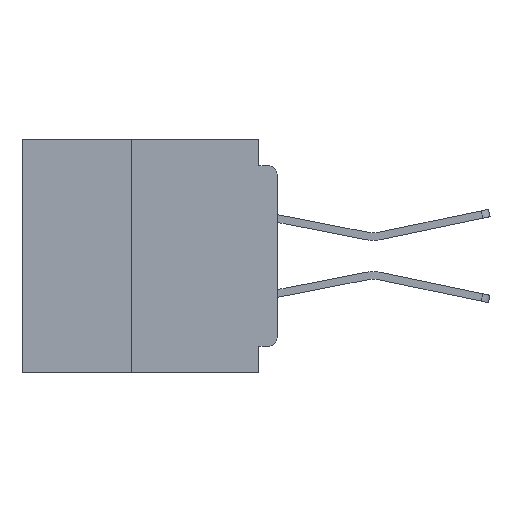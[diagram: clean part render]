
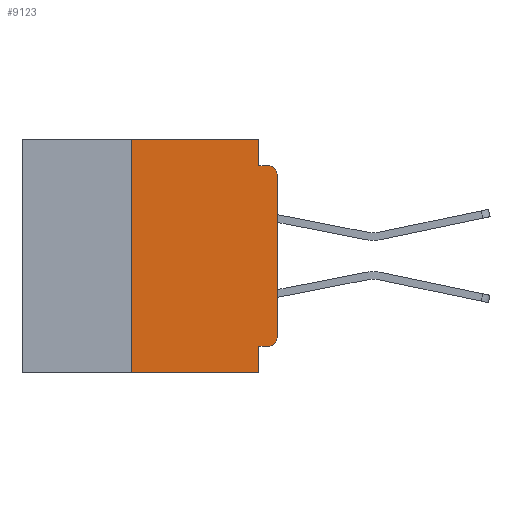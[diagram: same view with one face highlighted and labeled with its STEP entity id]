
A CAD part, left-side view. The second image highlights one B-rep face of the part: STEP entity #9123.
In plain terms, the highlighted planar face has unit normal (-1, 0, 0).
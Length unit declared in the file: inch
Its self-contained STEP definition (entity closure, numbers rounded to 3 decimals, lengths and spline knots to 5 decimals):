
#565 = VECTOR ( 'NONE', #24022, 39.37008 ) ;
#950 = EDGE_CURVE ( 'NONE', #38986, #4719, #29150, .T. ) ;
#1031 = CARTESIAN_POINT ( 'NONE',  ( 0., 0., -0.06 ) ) ;
#1445 = VECTOR ( 'NONE', #38640, 39.37008 ) ;
#2220 = VERTEX_POINT ( 'NONE', #16626 ) ;
#2329 = DIRECTION ( 'NONE',  ( 0., 0., -1. ) ) ;
#2563 = EDGE_CURVE ( 'NONE', #38383, #30484, #29532, .T. ) ;
#2853 = VECTOR ( 'NONE', #5867, 39.37008 ) ;
#4082 = EDGE_CURVE ( 'NONE', #17019, #30484, #7110, .T. ) ;
#4089 = VERTEX_POINT ( 'NONE', #6760 ) ;
#4719 = VERTEX_POINT ( 'NONE', #31256 ) ;
#5179 = CARTESIAN_POINT ( 'NONE',  ( 0., 0.25, -0.4 ) ) ;
#5496 = ORIENTED_EDGE ( 'NONE', *, *, #950, .T. ) ;
#5560 = VERTEX_POINT ( 'NONE', #18147 ) ;
#5867 = DIRECTION ( 'NONE',  ( 0., -1., 0. ) ) ;
#6497 = DIRECTION ( 'NONE',  ( 0., -1., 0. ) ) ;
#6699 = CARTESIAN_POINT ( 'NONE',  ( 0., 0., -0.045 ) ) ;
#6760 = CARTESIAN_POINT ( 'NONE',  ( 0., 0.015, -0.355 ) ) ;
#7110 = LINE ( 'NONE', #6699, #43730 ) ;
#7145 = ORIENTED_EDGE ( 'NONE', *, *, #4082, .F. ) ;
#8577 = ORIENTED_EDGE ( 'NONE', *, *, #44656, .F. ) ;
#9123 = ADVANCED_FACE ( 'NONE', ( #24068 ), #20915, .F. ) ;
#10241 = VECTOR ( 'NONE', #29576, 39.37008 ) ;
#11202 = CARTESIAN_POINT ( 'NONE',  ( 0., 0.031, -0.355 ) ) ;
#12438 = ORIENTED_EDGE ( 'NONE', *, *, #2563, .T. ) ;
#12932 = EDGE_CURVE ( 'NONE', #38986, #5560, #39465, .T. ) ;
#13228 = CARTESIAN_POINT ( 'NONE',  ( 0., 0.437, -0.4 ) ) ;
#13434 = CARTESIAN_POINT ( 'NONE',  ( 0., 0., 0. ) ) ;
#15357 = EDGE_CURVE ( 'NONE', #24697, #17019, #21614, .T. ) ;
#16626 = CARTESIAN_POINT ( 'NONE',  ( 0., 0., -0.34 ) ) ;
#16861 = ORIENTED_EDGE ( 'NONE', *, *, #28020, .T. ) ;
#16980 = EDGE_CURVE ( 'NONE', #4089, #44784, #19795, .T. ) ;
#17019 = VERTEX_POINT ( 'NONE', #43849 ) ;
#17351 = ORIENTED_EDGE ( 'NONE', *, *, #15357, .F. ) ;
#18147 = CARTESIAN_POINT ( 'NONE',  ( 0., 0.25, 0. ) ) ;
#18419 = CIRCLE ( 'NONE', #35934, 0.015 ) ;
#19558 = VECTOR ( 'NONE', #20291, 39.37008 ) ;
#19611 = EDGE_CURVE ( 'NONE', #5560, #24697, #29051, .T. ) ;
#19795 = LINE ( 'NONE', #22295, #10241 ) ;
#20291 = DIRECTION ( 'NONE',  ( 0., 0., 1. ) ) ;
#20442 = ORIENTED_EDGE ( 'NONE', *, *, #43913, .T. ) ;
#20915 = PLANE ( 'NONE',  #43250 ) ;
#21053 = DIRECTION ( 'NONE',  ( 1., 0., 0. ) ) ;
#21614 = LINE ( 'NONE', #45522, #1445 ) ;
#22295 = CARTESIAN_POINT ( 'NONE',  ( 0., 0., -0.355 ) ) ;
#22776 = VECTOR ( 'NONE', #42355, 39.37008 ) ;
#22968 = ORIENTED_EDGE ( 'NONE', *, *, #19611, .F. ) ;
#23734 = DIRECTION ( 'NONE',  ( -1., 0., 0. ) ) ;
#24022 = DIRECTION ( 'NONE',  ( 0., -1., 0. ) ) ;
#24068 = FACE_OUTER_BOUND ( 'NONE', #37482, .T. ) ;
#24269 = LINE ( 'NONE', #13434, #32581 ) ;
#24697 = VERTEX_POINT ( 'NONE', #34596 ) ;
#28020 = EDGE_CURVE ( 'NONE', #2220, #38383, #24269, .T. ) ;
#28346 = CARTESIAN_POINT ( 'NONE',  ( 0., 0.031, -0.4 ) ) ;
#28719 = ORIENTED_EDGE ( 'NONE', *, *, #12932, .F. ) ;
#29051 = LINE ( 'NONE', #41619, #565 ) ;
#29150 = LINE ( 'NONE', #13228, #2853 ) ;
#29532 = CIRCLE ( 'NONE', #43651, 0.015 ) ;
#29576 = DIRECTION ( 'NONE',  ( 0., 1., 0. ) ) ;
#30484 = VERTEX_POINT ( 'NONE', #42244 ) ;
#31256 = CARTESIAN_POINT ( 'NONE',  ( 0., 0.031, -0.4 ) ) ;
#32581 = VECTOR ( 'NONE', #34723, 39.37008 ) ;
#33295 = LINE ( 'NONE', #28346, #22776 ) ;
#34341 = CARTESIAN_POINT ( 'NONE',  ( 0., 0.25, -0.4 ) ) ;
#34596 = CARTESIAN_POINT ( 'NONE',  ( 0., 0.031, 0. ) ) ;
#34723 = DIRECTION ( 'NONE',  ( 0., 0., 1. ) ) ;
#35934 = AXIS2_PLACEMENT_3D ( 'NONE', #44819, #23734, #2329 ) ;
#37482 = EDGE_LOOP ( 'NONE', ( #16861, #12438, #7145, #17351, #22968, #28719, #5496, #8577, #38265, #20442 ) ) ;
#38265 = ORIENTED_EDGE ( 'NONE', *, *, #16980, .F. ) ;
#38383 = VERTEX_POINT ( 'NONE', #1031 ) ;
#38640 = DIRECTION ( 'NONE',  ( 0., 0., -1. ) ) ;
#38986 = VERTEX_POINT ( 'NONE', #5179 ) ;
#39465 = LINE ( 'NONE', #34341, #19558 ) ;
#41619 = CARTESIAN_POINT ( 'NONE',  ( 0., 0.437, 0. ) ) ;
#42196 = CARTESIAN_POINT ( 'NONE',  ( 0., 0.437, 0. ) ) ;
#42244 = CARTESIAN_POINT ( 'NONE',  ( 0., 0.015, -0.045 ) ) ;
#42355 = DIRECTION ( 'NONE',  ( 0., 0., -1. ) ) ;
#43250 = AXIS2_PLACEMENT_3D ( 'NONE', #42196, #21053, #45710 ) ;
#43651 = AXIS2_PLACEMENT_3D ( 'NONE', #43858, #43804, #43763 ) ;
#43730 = VECTOR ( 'NONE', #6497, 39.37008 ) ;
#43763 = DIRECTION ( 'NONE',  ( 0., 0., -1. ) ) ;
#43804 = DIRECTION ( 'NONE',  ( -1., 0., 0. ) ) ;
#43849 = CARTESIAN_POINT ( 'NONE',  ( 0., 0.031, -0.045 ) ) ;
#43858 = CARTESIAN_POINT ( 'NONE',  ( 0., 0.015, -0.06 ) ) ;
#43913 = EDGE_CURVE ( 'NONE', #4089, #2220, #18419, .T. ) ;
#44656 = EDGE_CURVE ( 'NONE', #44784, #4719, #33295, .T. ) ;
#44784 = VERTEX_POINT ( 'NONE', #11202 ) ;
#44819 = CARTESIAN_POINT ( 'NONE',  ( 0., 0.015, -0.34 ) ) ;
#45522 = CARTESIAN_POINT ( 'NONE',  ( 0., 0.031, 0. ) ) ;
#45710 = DIRECTION ( 'NONE',  ( 0., 0., -1. ) ) ;
